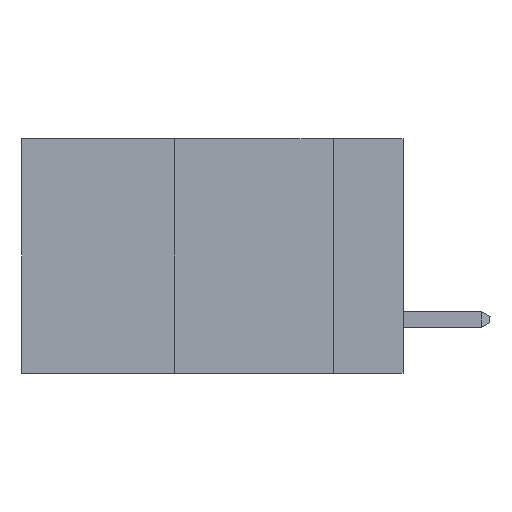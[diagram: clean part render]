
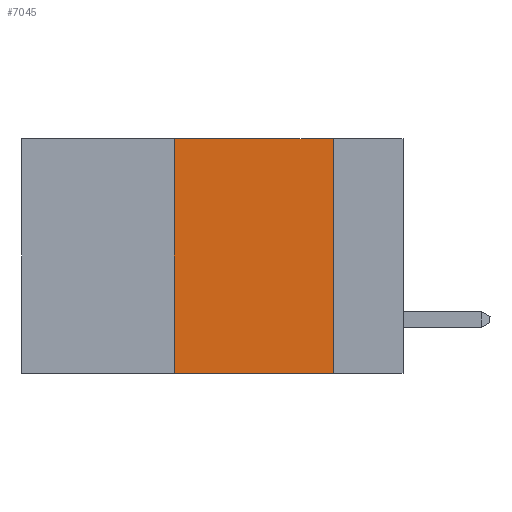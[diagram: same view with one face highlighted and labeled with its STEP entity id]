
A CAD part, left-side view. The second image highlights one B-rep face of the part: STEP entity #7045.
In plain terms, the highlighted planar face has unit normal (-1, 0, 0).
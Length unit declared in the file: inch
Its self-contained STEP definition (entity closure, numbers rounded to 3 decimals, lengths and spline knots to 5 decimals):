
#393 = VERTEX_POINT ( 'NONE', #3466 ) ;
#583 = VERTEX_POINT ( 'NONE', #6511 ) ;
#934 = VECTOR ( 'NONE', #12749, 39.37008 ) ;
#1142 = DIRECTION ( 'NONE',  ( 1., 0., 0. ) ) ;
#2364 = LINE ( 'NONE', #3339, #2832 ) ;
#2832 = VECTOR ( 'NONE', #3612, 39.37008 ) ;
#3074 = CARTESIAN_POINT ( 'NONE',  ( 0., 0.36, 0. ) ) ;
#3339 = CARTESIAN_POINT ( 'NONE',  ( 0., 0.6, 0. ) ) ;
#3394 = ORIENTED_EDGE ( 'NONE', *, *, #10836, .F. ) ;
#3466 = CARTESIAN_POINT ( 'NONE',  ( 0., 0.36, -0.37 ) ) ;
#3612 = DIRECTION ( 'NONE',  ( 0., -1., 0. ) ) ;
#3640 = DIRECTION ( 'NONE',  ( 0., -1., 0. ) ) ;
#4270 = DIRECTION ( 'NONE',  ( 0., 0., -1. ) ) ;
#4554 = LINE ( 'NONE', #5604, #9841 ) ;
#4701 = DIRECTION ( 'NONE',  ( 0., 0., -1. ) ) ;
#4716 = ORIENTED_EDGE ( 'NONE', *, *, #8621, .F. ) ;
#5512 = CARTESIAN_POINT ( 'NONE',  ( 0., 0.36, 0. ) ) ;
#5604 = CARTESIAN_POINT ( 'NONE',  ( 0., 0.6, -0.37 ) ) ;
#5746 = CARTESIAN_POINT ( 'NONE',  ( 0., 0.11, 0. ) ) ;
#5940 = VERTEX_POINT ( 'NONE', #5512 ) ;
#6341 = EDGE_CURVE ( 'NONE', #5940, #583, #2364, .T. ) ;
#6419 = VERTEX_POINT ( 'NONE', #6939 ) ;
#6511 = CARTESIAN_POINT ( 'NONE',  ( 0., 0.11, 0. ) ) ;
#6808 = AXIS2_PLACEMENT_3D ( 'NONE', #7116, #1142, #4270 ) ;
#6939 = CARTESIAN_POINT ( 'NONE',  ( 0., 0.11, -0.37 ) ) ;
#7045 = ADVANCED_FACE ( 'NONE', ( #12433 ), #7565, .F. ) ;
#7116 = CARTESIAN_POINT ( 'NONE',  ( 0., 0.6, 0. ) ) ;
#7351 = ORIENTED_EDGE ( 'NONE', *, *, #10563, .T. ) ;
#7494 = LINE ( 'NONE', #3074, #934 ) ;
#7565 = PLANE ( 'NONE',  #6808 ) ;
#7784 = LINE ( 'NONE', #5746, #9229 ) ;
#8259 = EDGE_LOOP ( 'NONE', ( #4716, #12217, #3394, #7351 ) ) ;
#8621 = EDGE_CURVE ( 'NONE', #583, #6419, #7784, .T. ) ;
#9229 = VECTOR ( 'NONE', #4701, 39.37008 ) ;
#9841 = VECTOR ( 'NONE', #3640, 39.37008 ) ;
#10563 = EDGE_CURVE ( 'NONE', #393, #6419, #4554, .T. ) ;
#10836 = EDGE_CURVE ( 'NONE', #393, #5940, #7494, .T. ) ;
#12217 = ORIENTED_EDGE ( 'NONE', *, *, #6341, .F. ) ;
#12433 = FACE_OUTER_BOUND ( 'NONE', #8259, .T. ) ;
#12749 = DIRECTION ( 'NONE',  ( 0., 0., 1. ) ) ;
